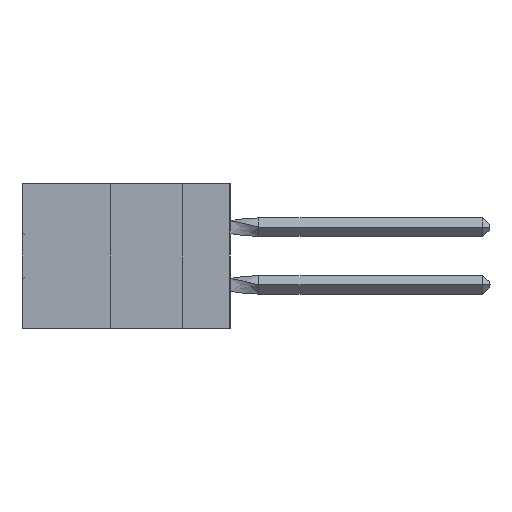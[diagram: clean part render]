
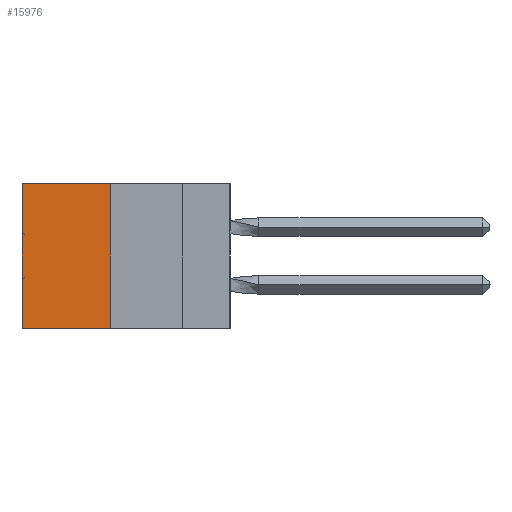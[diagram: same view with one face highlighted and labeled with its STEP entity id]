
A CAD part, left-side view. The second image highlights one B-rep face of the part: STEP entity #15976.
In plain terms, the highlighted planar face has unit normal (-1, 0, 0).
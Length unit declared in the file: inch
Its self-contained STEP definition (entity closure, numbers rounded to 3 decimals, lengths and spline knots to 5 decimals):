
#475 = DIRECTION ( 'NONE',  ( 0., 1., 0. ) ) ;
#4354 = EDGE_CURVE ( 'NONE', #41240, #4959, #40450, .T. ) ;
#4512 = FACE_OUTER_BOUND ( 'NONE', #24289, .T. ) ;
#4669 = LINE ( 'NONE', #17557, #39078 ) ;
#4959 = VERTEX_POINT ( 'NONE', #20664 ) ;
#7414 = DIRECTION ( 'NONE',  ( 1., 0., 0. ) ) ;
#10692 = EDGE_CURVE ( 'NONE', #20957, #52130, #21103, .T. ) ;
#11495 = DIRECTION ( 'NONE',  ( 0., 0., -1. ) ) ;
#11677 = PLANE ( 'NONE',  #13951 ) ;
#13951 = AXIS2_PLACEMENT_3D ( 'NONE', #31971, #7414, #11495 ) ;
#14592 = LINE ( 'NONE', #52631, #22266 ) ;
#14621 = EDGE_CURVE ( 'NONE', #4959, #52130, #4669, .T. ) ;
#15290 = CARTESIAN_POINT ( 'NONE',  ( 0.305, 0.413, -0.5 ) ) ;
#15976 = ADVANCED_FACE ( 'NONE', ( #4512 ), #11677, .F. ) ;
#17557 = CARTESIAN_POINT ( 'NONE',  ( 0.305, 0.413, -0.5 ) ) ;
#20664 = CARTESIAN_POINT ( 'NONE',  ( 0.305, 0.413, -0.5 ) ) ;
#20957 = VERTEX_POINT ( 'NONE', #27186 ) ;
#21018 = CARTESIAN_POINT ( 'NONE',  ( 0.305, 0.72, -0.5 ) ) ;
#21103 = LINE ( 'NONE', #21018, #31953 ) ;
#22266 = VECTOR ( 'NONE', #475, 39.37008 ) ;
#24289 = EDGE_LOOP ( 'NONE', ( #26226, #51387, #49344, #35741 ) ) ;
#26226 = ORIENTED_EDGE ( 'NONE', *, *, #10692, .T. ) ;
#27186 = CARTESIAN_POINT ( 'NONE',  ( 0.305, 0.72, 0. ) ) ;
#31953 = VECTOR ( 'NONE', #33338, 39.37008 ) ;
#31971 = CARTESIAN_POINT ( 'NONE',  ( 0.305, 0.413, -0.5 ) ) ;
#33338 = DIRECTION ( 'NONE',  ( 0., 0., -1. ) ) ;
#34603 = CARTESIAN_POINT ( 'NONE',  ( 0.305, 0.413, 0. ) ) ;
#35141 = DIRECTION ( 'NONE',  ( 0., 0., -1. ) ) ;
#35741 = ORIENTED_EDGE ( 'NONE', *, *, #43503, .T. ) ;
#39078 = VECTOR ( 'NONE', #50721, 39.37008 ) ;
#40450 = LINE ( 'NONE', #15290, #48696 ) ;
#41240 = VERTEX_POINT ( 'NONE', #34603 ) ;
#43503 = EDGE_CURVE ( 'NONE', #41240, #20957, #14592, .T. ) ;
#48596 = CARTESIAN_POINT ( 'NONE',  ( 0.305, 0.72, -0.5 ) ) ;
#48696 = VECTOR ( 'NONE', #35141, 39.37008 ) ;
#49344 = ORIENTED_EDGE ( 'NONE', *, *, #4354, .F. ) ;
#50721 = DIRECTION ( 'NONE',  ( 0., 1., 0. ) ) ;
#51387 = ORIENTED_EDGE ( 'NONE', *, *, #14621, .F. ) ;
#52130 = VERTEX_POINT ( 'NONE', #48596 ) ;
#52631 = CARTESIAN_POINT ( 'NONE',  ( 0.305, 0.413, 0. ) ) ;
